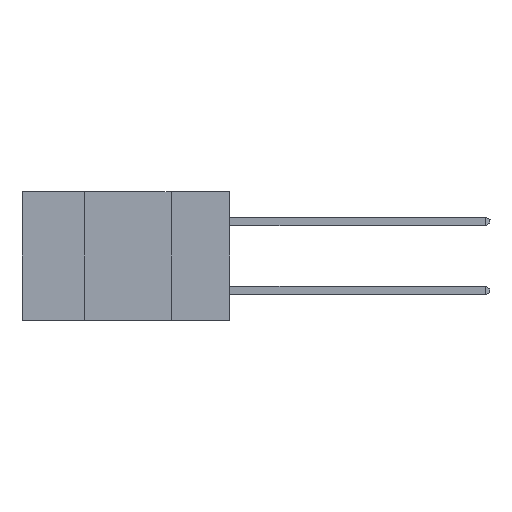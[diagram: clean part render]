
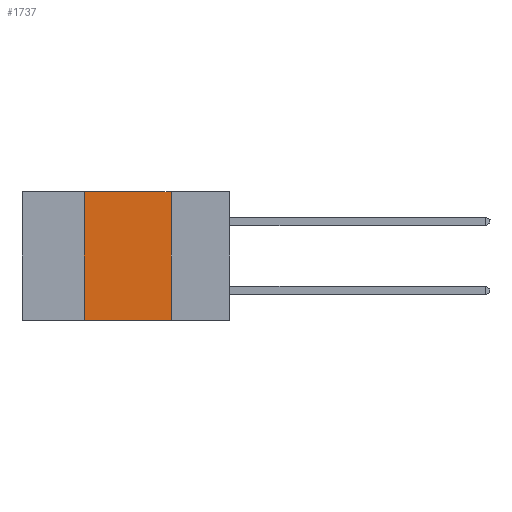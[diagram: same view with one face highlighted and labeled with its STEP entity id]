
A CAD part, left-side view. The second image highlights one B-rep face of the part: STEP entity #1737.
In plain terms, the highlighted planar face has unit normal (-1, 0, 0).
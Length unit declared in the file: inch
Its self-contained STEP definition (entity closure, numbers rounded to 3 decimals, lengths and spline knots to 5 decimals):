
#84 = DIRECTION ( 'NONE',  ( 0., 0., 1. ) ) ;
#352 = CARTESIAN_POINT ( 'NONE',  ( 0., 0.17, 0. ) ) ;
#529 = AXIS2_PLACEMENT_3D ( 'NONE', #21469, #1574, #1567 ) ;
#1356 = EDGE_CURVE ( 'NONE', #22014, #2103, #12008, .T. ) ;
#1567 = DIRECTION ( 'NONE',  ( 0., 0., -1. ) ) ;
#1574 = DIRECTION ( 'NONE',  ( 1., 0., 0. ) ) ;
#1596 = PLANE ( 'NONE',  #529 ) ;
#1737 = ADVANCED_FACE ( 'NONE', ( #21051 ), #1596, .F. ) ;
#2103 = VERTEX_POINT ( 'NONE', #5298 ) ;
#2467 = VERTEX_POINT ( 'NONE', #352 ) ;
#3659 = EDGE_LOOP ( 'NONE', ( #15591, #17667, #18133, #16547 ) ) ;
#4860 = DIRECTION ( 'NONE',  ( 0., 0., -1. ) ) ;
#5298 = CARTESIAN_POINT ( 'NONE',  ( 0., 0.42, 0. ) ) ;
#5952 = LINE ( 'NONE', #5995, #14988 ) ;
#5995 = CARTESIAN_POINT ( 'NONE',  ( 0., 0.6, -0.37 ) ) ;
#8292 = CARTESIAN_POINT ( 'NONE',  ( 0., 0.6, 0. ) ) ;
#8530 = CARTESIAN_POINT ( 'NONE',  ( 0., 0.42, 0. ) ) ;
#8592 = CARTESIAN_POINT ( 'NONE',  ( 0., 0.17, -0.37 ) ) ;
#8730 = LINE ( 'NONE', #21927, #12752 ) ;
#10018 = DIRECTION ( 'NONE',  ( 0., -1., 0. ) ) ;
#12008 = LINE ( 'NONE', #8530, #21069 ) ;
#12265 = CARTESIAN_POINT ( 'NONE',  ( 0., 0.42, -0.37 ) ) ;
#12404 = EDGE_CURVE ( 'NONE', #22014, #15305, #5952, .T. ) ;
#12752 = VECTOR ( 'NONE', #4860, 39.37008 ) ;
#14988 = VECTOR ( 'NONE', #16191, 39.37008 ) ;
#15305 = VERTEX_POINT ( 'NONE', #8592 ) ;
#15591 = ORIENTED_EDGE ( 'NONE', *, *, #21841, .F. ) ;
#15990 = VECTOR ( 'NONE', #10018, 39.37008 ) ;
#16191 = DIRECTION ( 'NONE',  ( 0., -1., 0. ) ) ;
#16547 = ORIENTED_EDGE ( 'NONE', *, *, #12404, .T. ) ;
#17667 = ORIENTED_EDGE ( 'NONE', *, *, #18942, .F. ) ;
#18133 = ORIENTED_EDGE ( 'NONE', *, *, #1356, .F. ) ;
#18942 = EDGE_CURVE ( 'NONE', #2103, #2467, #20519, .T. ) ;
#20519 = LINE ( 'NONE', #8292, #15990 ) ;
#21051 = FACE_OUTER_BOUND ( 'NONE', #3659, .T. ) ;
#21069 = VECTOR ( 'NONE', #84, 39.37008 ) ;
#21469 = CARTESIAN_POINT ( 'NONE',  ( 0., 0.6, 0. ) ) ;
#21841 = EDGE_CURVE ( 'NONE', #2467, #15305, #8730, .T. ) ;
#21927 = CARTESIAN_POINT ( 'NONE',  ( 0., 0.17, 0. ) ) ;
#22014 = VERTEX_POINT ( 'NONE', #12265 ) ;
